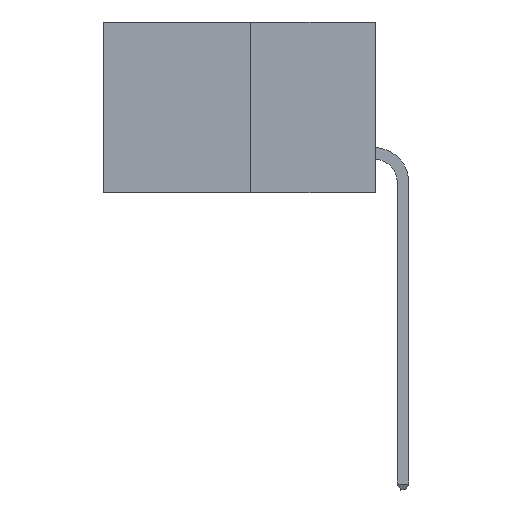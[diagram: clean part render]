
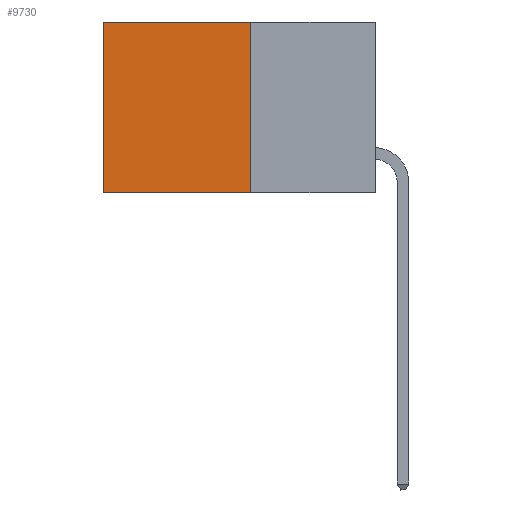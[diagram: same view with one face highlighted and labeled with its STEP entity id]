
A CAD part, left-side view. The second image highlights one B-rep face of the part: STEP entity #9730.
In plain terms, the highlighted planar face has unit normal (-1, 0, 0).
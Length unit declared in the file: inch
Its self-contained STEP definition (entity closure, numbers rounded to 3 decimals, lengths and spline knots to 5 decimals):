
#12 = EDGE_CURVE ( 'NONE', #24016, #23914, #15867, .T. ) ;
#175 = CARTESIAN_POINT ( 'NONE',  ( 0.277, 0.27, 0. ) ) ;
#1408 = EDGE_CURVE ( 'NONE', #23914, #17944, #19118, .T. ) ;
#2202 = ORIENTED_EDGE ( 'NONE', *, *, #1408, .T. ) ;
#2378 = LINE ( 'NONE', #9660, #11472 ) ;
#3374 = CARTESIAN_POINT ( 'NONE',  ( 0.277, 0.27, -0.37 ) ) ;
#4095 = CARTESIAN_POINT ( 'NONE',  ( 0.277, 0.27, -0.37 ) ) ;
#4435 = VERTEX_POINT ( 'NONE', #4095 ) ;
#6786 = ORIENTED_EDGE ( 'NONE', *, *, #15178, .F. ) ;
#7330 = DIRECTION ( 'NONE',  ( 0., 0., -1. ) ) ;
#8688 = DIRECTION ( 'NONE',  ( 0., 1., 0. ) ) ;
#9061 = CARTESIAN_POINT ( 'NONE',  ( 0.277, 0.59, -0.37 ) ) ;
#9115 = PLANE ( 'NONE',  #13040 ) ;
#9660 = CARTESIAN_POINT ( 'NONE',  ( 0.277, 0.27, -0.37 ) ) ;
#9730 = ADVANCED_FACE ( 'NONE', ( #13742 ), #9115, .F. ) ;
#10213 = VECTOR ( 'NONE', #8688, 39.37008 ) ;
#10427 = CARTESIAN_POINT ( 'NONE',  ( 0.277, 0.59, 0. ) ) ;
#10681 = CARTESIAN_POINT ( 'NONE',  ( 0.277, 0.27, 0. ) ) ;
#11057 = DIRECTION ( 'NONE',  ( 0., 0., -1. ) ) ;
#11472 = VECTOR ( 'NONE', #7330, 39.37008 ) ;
#11972 = VECTOR ( 'NONE', #13045, 39.37008 ) ;
#13040 = AXIS2_PLACEMENT_3D ( 'NONE', #14733, #22495, #11057 ) ;
#13045 = DIRECTION ( 'NONE',  ( 0., 1., 0. ) ) ;
#13742 = FACE_OUTER_BOUND ( 'NONE', #15892, .T. ) ;
#13976 = VECTOR ( 'NONE', #20783, 39.37008 ) ;
#14733 = CARTESIAN_POINT ( 'NONE',  ( 0.277, 0.27, -0.37 ) ) ;
#15178 = EDGE_CURVE ( 'NONE', #24016, #4435, #2378, .T. ) ;
#15867 = LINE ( 'NONE', #175, #10213 ) ;
#15892 = EDGE_LOOP ( 'NONE', ( #2202, #19065, #6786, #24590 ) ) ;
#17041 = LINE ( 'NONE', #3374, #11972 ) ;
#17944 = VERTEX_POINT ( 'NONE', #23103 ) ;
#19065 = ORIENTED_EDGE ( 'NONE', *, *, #20460, .F. ) ;
#19118 = LINE ( 'NONE', #9061, #13976 ) ;
#20460 = EDGE_CURVE ( 'NONE', #4435, #17944, #17041, .T. ) ;
#20783 = DIRECTION ( 'NONE',  ( 0., 0., -1. ) ) ;
#22495 = DIRECTION ( 'NONE',  ( 1., 0., 0. ) ) ;
#23103 = CARTESIAN_POINT ( 'NONE',  ( 0.277, 0.59, -0.37 ) ) ;
#23914 = VERTEX_POINT ( 'NONE', #10427 ) ;
#24016 = VERTEX_POINT ( 'NONE', #10681 ) ;
#24590 = ORIENTED_EDGE ( 'NONE', *, *, #12, .T. ) ;
